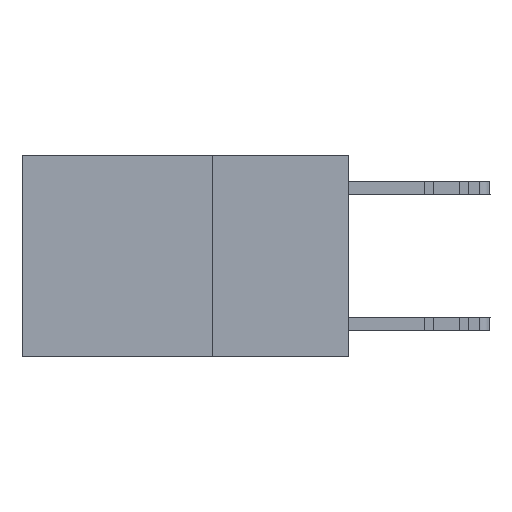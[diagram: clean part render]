
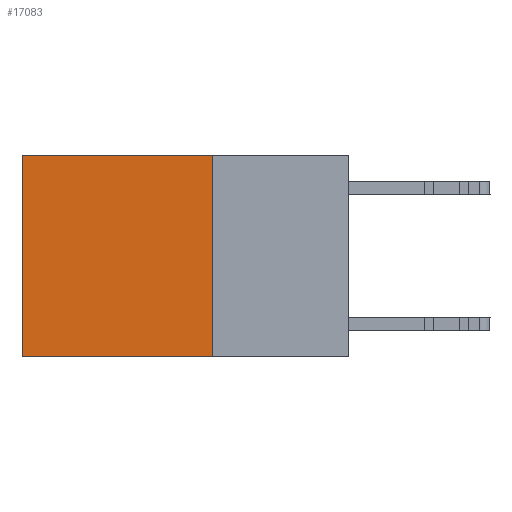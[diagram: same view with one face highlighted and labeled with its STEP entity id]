
A CAD part, left-side view. The second image highlights one B-rep face of the part: STEP entity #17083.
In plain terms, the highlighted planar face has unit normal (-1, 0, 0).
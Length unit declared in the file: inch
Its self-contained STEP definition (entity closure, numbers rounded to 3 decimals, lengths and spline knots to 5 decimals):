
#159 = ORIENTED_EDGE ( 'NONE', *, *, #25241, .T. ) ;
#502 = VECTOR ( 'NONE', #27726, 39.37008 ) ;
#629 = LINE ( 'NONE', #27686, #502 ) ;
#1279 = DIRECTION ( 'NONE',  ( 0., 1., 0. ) ) ;
#1495 = CARTESIAN_POINT ( 'NONE',  ( 0.2625, 0.25, -0.37 ) ) ;
#2901 = EDGE_CURVE ( 'NONE', #14925, #16658, #6254, .T. ) ;
#4913 = FACE_OUTER_BOUND ( 'NONE', #19010, .T. ) ;
#6230 = VECTOR ( 'NONE', #8962, 39.37008 ) ;
#6254 = LINE ( 'NONE', #12691, #6230 ) ;
#7647 = DIRECTION ( 'NONE',  ( 0., 0., -1. ) ) ;
#7714 = DIRECTION ( 'NONE',  ( 1., 0., 0. ) ) ;
#7754 = CARTESIAN_POINT ( 'NONE',  ( 0.2625, 0.25, 0. ) ) ;
#7880 = PLANE ( 'NONE',  #24808 ) ;
#8818 = VERTEX_POINT ( 'NONE', #9406 ) ;
#8962 = DIRECTION ( 'NONE',  ( 0., 0., -1. ) ) ;
#9406 = CARTESIAN_POINT ( 'NONE',  ( 0.2625, 0.25, 0. ) ) ;
#11321 = CARTESIAN_POINT ( 'NONE',  ( 0.2625, 0.6, 0. ) ) ;
#11922 = VERTEX_POINT ( 'NONE', #21843 ) ;
#12530 = VECTOR ( 'NONE', #28394, 39.37008 ) ;
#12673 = EDGE_CURVE ( 'NONE', #8818, #11922, #629, .T. ) ;
#12691 = CARTESIAN_POINT ( 'NONE',  ( 0.2625, 0.6, 0. ) ) ;
#14559 = ORIENTED_EDGE ( 'NONE', *, *, #2901, .T. ) ;
#14925 = VERTEX_POINT ( 'NONE', #11321 ) ;
#15538 = CARTESIAN_POINT ( 'NONE',  ( 0.2625, 0.6, -0.37 ) ) ;
#15567 = VECTOR ( 'NONE', #1279, 39.37008 ) ;
#16658 = VERTEX_POINT ( 'NONE', #15538 ) ;
#17083 = ADVANCED_FACE ( 'NONE', ( #4913 ), #7880, .F. ) ;
#19010 = EDGE_LOOP ( 'NONE', ( #14559, #19672, #27233, #159 ) ) ;
#19672 = ORIENTED_EDGE ( 'NONE', *, *, #25290, .F. ) ;
#21843 = CARTESIAN_POINT ( 'NONE',  ( 0.2625, 0.25, -0.37 ) ) ;
#24808 = AXIS2_PLACEMENT_3D ( 'NONE', #7754, #7714, #7647 ) ;
#25241 = EDGE_CURVE ( 'NONE', #8818, #14925, #28426, .T. ) ;
#25290 = EDGE_CURVE ( 'NONE', #11922, #16658, #26205, .T. ) ;
#26205 = LINE ( 'NONE', #1495, #12530 ) ;
#27233 = ORIENTED_EDGE ( 'NONE', *, *, #12673, .F. ) ;
#27686 = CARTESIAN_POINT ( 'NONE',  ( 0.2625, 0.25, 0. ) ) ;
#27726 = DIRECTION ( 'NONE',  ( 0., 0., -1. ) ) ;
#28394 = DIRECTION ( 'NONE',  ( 0., 1., 0. ) ) ;
#28426 = LINE ( 'NONE', #30579, #15567 ) ;
#30579 = CARTESIAN_POINT ( 'NONE',  ( 0.2625, 0.25, 0. ) ) ;
